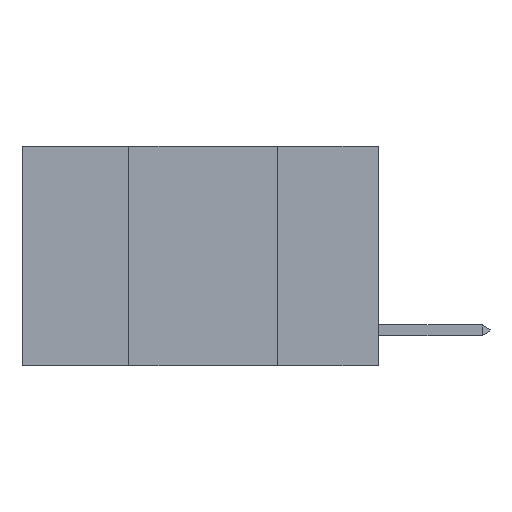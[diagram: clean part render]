
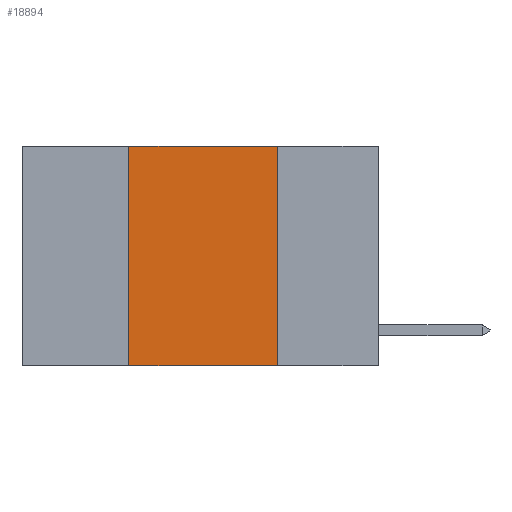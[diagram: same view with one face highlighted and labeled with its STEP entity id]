
A CAD part, left-side view. The second image highlights one B-rep face of the part: STEP entity #18894.
In plain terms, the highlighted planar face has unit normal (-1, 0, 0).
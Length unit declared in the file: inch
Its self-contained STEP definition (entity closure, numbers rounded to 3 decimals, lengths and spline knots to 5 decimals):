
#1098 = VERTEX_POINT ( 'NONE', #19685 ) ;
#1877 = AXIS2_PLACEMENT_3D ( 'NONE', #16402, #18093, #7920 ) ;
#2116 = CARTESIAN_POINT ( 'NONE',  ( 0., 0.42, -0.37 ) ) ;
#2169 = LINE ( 'NONE', #17928, #19097 ) ;
#3873 = EDGE_CURVE ( 'NONE', #15091, #9064, #8532, .T. ) ;
#4645 = EDGE_CURVE ( 'NONE', #1098, #13996, #2169, .T. ) ;
#5203 = ORIENTED_EDGE ( 'NONE', *, *, #20033, .F. ) ;
#5861 = LINE ( 'NONE', #6133, #14311 ) ;
#6133 = CARTESIAN_POINT ( 'NONE',  ( 0., 0.6, 0. ) ) ;
#6249 = PLANE ( 'NONE',  #1877 ) ;
#7706 = CARTESIAN_POINT ( 'NONE',  ( 0., 0.42, 0. ) ) ;
#7920 = DIRECTION ( 'NONE',  ( 0., 0., -1. ) ) ;
#8532 = LINE ( 'NONE', #17598, #12507 ) ;
#9064 = VERTEX_POINT ( 'NONE', #7706 ) ;
#9711 = CARTESIAN_POINT ( 'NONE',  ( 0., 0.17, -0.37 ) ) ;
#10672 = EDGE_CURVE ( 'NONE', #15091, #13996, #18645, .T. ) ;
#11187 = DIRECTION ( 'NONE',  ( 0., -1., 0. ) ) ;
#11727 = ORIENTED_EDGE ( 'NONE', *, *, #4645, .F. ) ;
#12507 = VECTOR ( 'NONE', #15986, 39.37008 ) ;
#13878 = ORIENTED_EDGE ( 'NONE', *, *, #3873, .F. ) ;
#13996 = VERTEX_POINT ( 'NONE', #9711 ) ;
#14311 = VECTOR ( 'NONE', #16298, 39.37008 ) ;
#15091 = VERTEX_POINT ( 'NONE', #2116 ) ;
#15986 = DIRECTION ( 'NONE',  ( 0., 0., 1. ) ) ;
#16298 = DIRECTION ( 'NONE',  ( 0., -1., 0. ) ) ;
#16402 = CARTESIAN_POINT ( 'NONE',  ( 0., 0.6, 0. ) ) ;
#17598 = CARTESIAN_POINT ( 'NONE',  ( 0., 0.42, 0. ) ) ;
#17904 = CARTESIAN_POINT ( 'NONE',  ( 0., 0.6, -0.37 ) ) ;
#17928 = CARTESIAN_POINT ( 'NONE',  ( 0., 0.17, 0. ) ) ;
#18093 = DIRECTION ( 'NONE',  ( 1., 0., 0. ) ) ;
#18645 = LINE ( 'NONE', #17904, #19175 ) ;
#18894 = ADVANCED_FACE ( 'NONE', ( #20231 ), #6249, .F. ) ;
#19097 = VECTOR ( 'NONE', #21360, 39.37008 ) ;
#19175 = VECTOR ( 'NONE', #11187, 39.37008 ) ;
#19662 = ORIENTED_EDGE ( 'NONE', *, *, #10672, .T. ) ;
#19685 = CARTESIAN_POINT ( 'NONE',  ( 0., 0.17, 0. ) ) ;
#20033 = EDGE_CURVE ( 'NONE', #9064, #1098, #5861, .T. ) ;
#20231 = FACE_OUTER_BOUND ( 'NONE', #21435, .T. ) ;
#21360 = DIRECTION ( 'NONE',  ( 0., 0., -1. ) ) ;
#21435 = EDGE_LOOP ( 'NONE', ( #11727, #5203, #13878, #19662 ) ) ;
